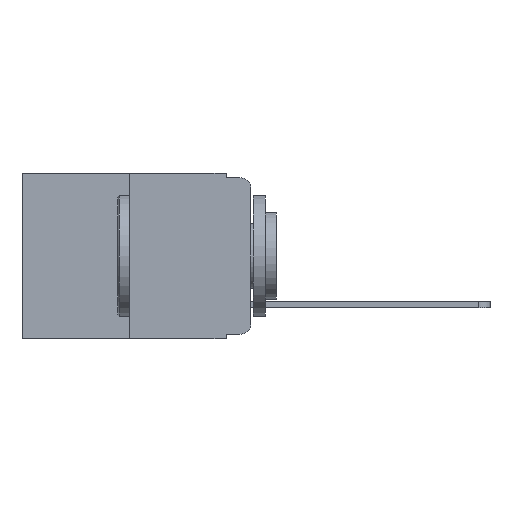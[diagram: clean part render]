
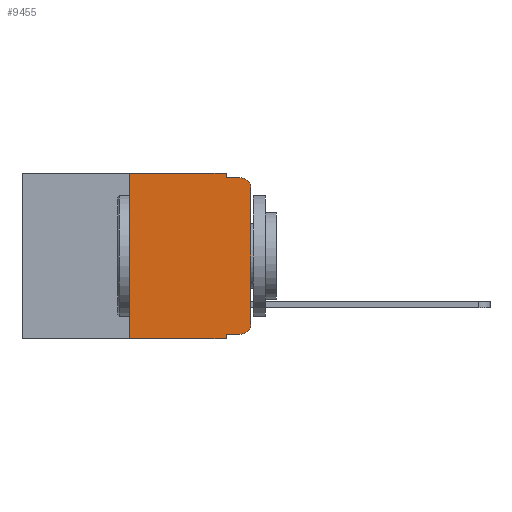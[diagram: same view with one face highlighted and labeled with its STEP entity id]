
A CAD part, left-side view. The second image highlights one B-rep face of the part: STEP entity #9455.
In plain terms, the highlighted planar face has unit normal (-1, 0, 0).
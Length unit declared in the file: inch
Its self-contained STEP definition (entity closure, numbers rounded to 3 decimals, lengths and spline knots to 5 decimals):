
#166 = VERTEX_POINT ( 'NONE', #9585 ) ;
#168 = DIRECTION ( 'NONE',  ( 0., 0., -1. ) ) ;
#253 = EDGE_CURVE ( 'NONE', #7558, #3400, #17359, .T. ) ;
#1101 = CARTESIAN_POINT ( 'NONE',  ( 0., 0.02, -0.03 ) ) ;
#1202 = CARTESIAN_POINT ( 'NONE',  ( 0., 0.051, -0.01 ) ) ;
#1306 = EDGE_CURVE ( 'NONE', #8923, #14996, #2503, .T. ) ;
#1482 = VECTOR ( 'NONE', #18921, 39.37008 ) ;
#1543 = CIRCLE ( 'NONE', #9276, 0.02 ) ;
#2136 = CARTESIAN_POINT ( 'NONE',  ( 0., 0., 0. ) ) ;
#2316 = CARTESIAN_POINT ( 'NONE',  ( 0., 0.473, 0. ) ) ;
#2503 = LINE ( 'NONE', #2136, #13535 ) ;
#2975 = AXIS2_PLACEMENT_3D ( 'NONE', #3744, #6626, #3678 ) ;
#3044 = VECTOR ( 'NONE', #8385, 39.37008 ) ;
#3400 = VERTEX_POINT ( 'NONE', #15651 ) ;
#3564 = CARTESIAN_POINT ( 'NONE',  ( 0., 0.02, -0.313 ) ) ;
#3678 = DIRECTION ( 'NONE',  ( 0., 0., -1. ) ) ;
#3710 = ORIENTED_EDGE ( 'NONE', *, *, #9850, .F. ) ;
#3744 = CARTESIAN_POINT ( 'NONE',  ( 0., 0.473, 0. ) ) ;
#4206 = EDGE_CURVE ( 'NONE', #3400, #8923, #5317, .T. ) ;
#4360 = EDGE_LOOP ( 'NONE', ( #14326, #6809, #10156, #7653, #9459, #3710, #10578, #8440, #11609, #15194 ) ) ;
#4666 = DIRECTION ( 'NONE',  ( 0., 0., -1. ) ) ;
#4838 = LINE ( 'NONE', #17443, #19371 ) ;
#5063 = DIRECTION ( 'NONE',  ( -1., 0., 0. ) ) ;
#5317 = CIRCLE ( 'NONE', #11242, 0.02 ) ;
#5590 = VERTEX_POINT ( 'NONE', #15086 ) ;
#6156 = EDGE_CURVE ( 'NONE', #166, #8347, #16522, .T. ) ;
#6162 = VECTOR ( 'NONE', #4666, 39.37008 ) ;
#6352 = CARTESIAN_POINT ( 'NONE',  ( 0., 0.051, -0.333 ) ) ;
#6626 = DIRECTION ( 'NONE',  ( 1., 0., 0. ) ) ;
#6809 = ORIENTED_EDGE ( 'NONE', *, *, #8643, .T. ) ;
#6882 = DIRECTION ( 'NONE',  ( -1., 0., 0. ) ) ;
#7558 = VERTEX_POINT ( 'NONE', #7835 ) ;
#7653 = ORIENTED_EDGE ( 'NONE', *, *, #13525, .F. ) ;
#7835 = CARTESIAN_POINT ( 'NONE',  ( 0., 0.051, -0.333 ) ) ;
#7837 = DIRECTION ( 'NONE',  ( 0., -1., 0. ) ) ;
#8347 = VERTEX_POINT ( 'NONE', #13704 ) ;
#8385 = DIRECTION ( 'NONE',  ( 0., -1., 0. ) ) ;
#8440 = ORIENTED_EDGE ( 'NONE', *, *, #19338, .F. ) ;
#8617 = EDGE_CURVE ( 'NONE', #14887, #5590, #4838, .T. ) ;
#8643 = EDGE_CURVE ( 'NONE', #14996, #5590, #1543, .T. ) ;
#8923 = VERTEX_POINT ( 'NONE', #13618 ) ;
#9161 = CARTESIAN_POINT ( 'NONE',  ( 0., 0.051, 0. ) ) ;
#9276 = AXIS2_PLACEMENT_3D ( 'NONE', #1101, #6882, #16476 ) ;
#9455 = ADVANCED_FACE ( 'NONE', ( #12286 ), #17256, .F. ) ;
#9459 = ORIENTED_EDGE ( 'NONE', *, *, #17945, .F. ) ;
#9568 = CARTESIAN_POINT ( 'NONE',  ( 0., 0.051, 0. ) ) ;
#9585 = CARTESIAN_POINT ( 'NONE',  ( 0., 0.25, -0.343 ) ) ;
#9850 = EDGE_CURVE ( 'NONE', #166, #13407, #14400, .T. ) ;
#10156 = ORIENTED_EDGE ( 'NONE', *, *, #8617, .F. ) ;
#10325 = CARTESIAN_POINT ( 'NONE',  ( 0., 0., -0.03 ) ) ;
#10578 = ORIENTED_EDGE ( 'NONE', *, *, #6156, .T. ) ;
#11242 = AXIS2_PLACEMENT_3D ( 'NONE', #3564, #5063, #11551 ) ;
#11551 = DIRECTION ( 'NONE',  ( 0., 0., -1. ) ) ;
#11609 = ORIENTED_EDGE ( 'NONE', *, *, #253, .T. ) ;
#11618 = CARTESIAN_POINT ( 'NONE',  ( 0., 0.25, 0. ) ) ;
#11958 = LINE ( 'NONE', #2316, #3044 ) ;
#12286 = FACE_OUTER_BOUND ( 'NONE', #4360, .T. ) ;
#12629 = DIRECTION ( 'NONE',  ( 0., 0., 1. ) ) ;
#13407 = VERTEX_POINT ( 'NONE', #11618 ) ;
#13525 = EDGE_CURVE ( 'NONE', #16759, #14887, #18844, .T. ) ;
#13535 = VECTOR ( 'NONE', #12629, 39.37008 ) ;
#13618 = CARTESIAN_POINT ( 'NONE',  ( 0., 0., -0.313 ) ) ;
#13641 = CARTESIAN_POINT ( 'NONE',  ( 0., 0.051, 0. ) ) ;
#13704 = CARTESIAN_POINT ( 'NONE',  ( 0., 0.051, -0.343 ) ) ;
#14326 = ORIENTED_EDGE ( 'NONE', *, *, #1306, .T. ) ;
#14400 = LINE ( 'NONE', #18081, #14651 ) ;
#14651 = VECTOR ( 'NONE', #16720, 39.37008 ) ;
#14887 = VERTEX_POINT ( 'NONE', #1202 ) ;
#14996 = VERTEX_POINT ( 'NONE', #10325 ) ;
#15086 = CARTESIAN_POINT ( 'NONE',  ( 0., 0.02, -0.01 ) ) ;
#15194 = ORIENTED_EDGE ( 'NONE', *, *, #4206, .T. ) ;
#15651 = CARTESIAN_POINT ( 'NONE',  ( 0., 0.02, -0.333 ) ) ;
#15668 = LINE ( 'NONE', #9161, #19398 ) ;
#15879 = DIRECTION ( 'NONE',  ( 0., -1., 0. ) ) ;
#15953 = VECTOR ( 'NONE', #7837, 39.37008 ) ;
#16476 = DIRECTION ( 'NONE',  ( 0., 0., -1. ) ) ;
#16522 = LINE ( 'NONE', #19172, #1482 ) ;
#16720 = DIRECTION ( 'NONE',  ( 0., 0., 1. ) ) ;
#16759 = VERTEX_POINT ( 'NONE', #9568 ) ;
#17256 = PLANE ( 'NONE',  #2975 ) ;
#17359 = LINE ( 'NONE', #6352, #15953 ) ;
#17443 = CARTESIAN_POINT ( 'NONE',  ( 0., 0.051, -0.01 ) ) ;
#17945 = EDGE_CURVE ( 'NONE', #13407, #16759, #11958, .T. ) ;
#18081 = CARTESIAN_POINT ( 'NONE',  ( 0., 0.25, 0. ) ) ;
#18844 = LINE ( 'NONE', #13641, #6162 ) ;
#18921 = DIRECTION ( 'NONE',  ( 0., -1., 0. ) ) ;
#19172 = CARTESIAN_POINT ( 'NONE',  ( 0., 0.473, -0.343 ) ) ;
#19338 = EDGE_CURVE ( 'NONE', #7558, #8347, #15668, .T. ) ;
#19371 = VECTOR ( 'NONE', #15879, 39.37008 ) ;
#19398 = VECTOR ( 'NONE', #168, 39.37008 ) ;
